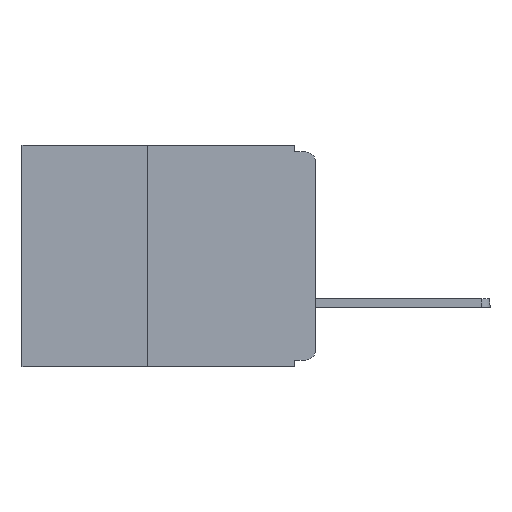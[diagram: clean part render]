
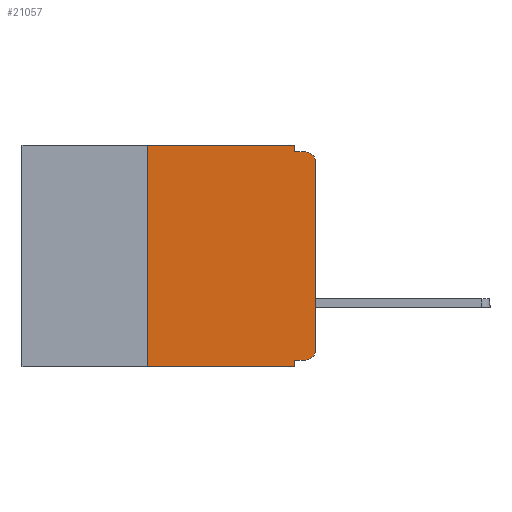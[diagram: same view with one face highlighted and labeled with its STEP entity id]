
A CAD part, left-side view. The second image highlights one B-rep face of the part: STEP entity #21057.
In plain terms, the highlighted planar face has unit normal (-1, 0, 0).
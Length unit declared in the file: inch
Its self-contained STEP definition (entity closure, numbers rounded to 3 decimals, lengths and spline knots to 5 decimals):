
#361 = VECTOR ( 'NONE', #23522, 39.37008 ) ;
#464 = VECTOR ( 'NONE', #29746, 39.37008 ) ;
#555 = DIRECTION ( 'NONE',  ( 0., 0., -1. ) ) ;
#592 = LINE ( 'NONE', #11071, #14531 ) ;
#637 = AXIS2_PLACEMENT_3D ( 'NONE', #30799, #15090, #33387 ) ;
#917 = ORIENTED_EDGE ( 'NONE', *, *, #19872, .F. ) ;
#2514 = ORIENTED_EDGE ( 'NONE', *, *, #29880, .F. ) ;
#3425 = VERTEX_POINT ( 'NONE', #17039 ) ;
#4144 = EDGE_CURVE ( 'NONE', #6339, #31770, #23790, .T. ) ;
#4825 = CARTESIAN_POINT ( 'NONE',  ( 0., 0., -0.305 ) ) ;
#5319 = CARTESIAN_POINT ( 'NONE',  ( 0., 0.437, 0. ) ) ;
#5727 = VERTEX_POINT ( 'NONE', #18445 ) ;
#5897 = CARTESIAN_POINT ( 'NONE',  ( 0., 0.031, 0. ) ) ;
#6339 = VERTEX_POINT ( 'NONE', #23707 ) ;
#6454 = EDGE_CURVE ( 'NONE', #5727, #31805, #20805, .T. ) ;
#6858 = EDGE_LOOP ( 'NONE', ( #20339, #23493, #17405, #27583, #917, #2514, #21348, #10965, #12615, #20300 ) ) ;
#7331 = DIRECTION ( 'NONE',  ( 1., 0., 0. ) ) ;
#7677 = EDGE_CURVE ( 'NONE', #17097, #15814, #9293, .T. ) ;
#7737 = DIRECTION ( 'NONE',  ( 0., 0., 1. ) ) ;
#7818 = CARTESIAN_POINT ( 'NONE',  ( 0., 0.015, -0.305 ) ) ;
#8336 = EDGE_CURVE ( 'NONE', #17097, #5727, #10124, .T. ) ;
#9293 = CIRCLE ( 'NONE', #22206, 0.015 ) ;
#9300 = VECTOR ( 'NONE', #18273, 39.37008 ) ;
#9304 = CARTESIAN_POINT ( 'NONE',  ( 0., 0.015, -0.32 ) ) ;
#9521 = VECTOR ( 'NONE', #12684, 39.37008 ) ;
#10124 = LINE ( 'NONE', #28785, #9300 ) ;
#10361 = VECTOR ( 'NONE', #14296, 39.37008 ) ;
#10410 = CARTESIAN_POINT ( 'NONE',  ( 0., 0.031, -0.33 ) ) ;
#10469 = DIRECTION ( 'NONE',  ( 0., 0., -1. ) ) ;
#10944 = EDGE_CURVE ( 'NONE', #15395, #16290, #21357, .T. ) ;
#10961 = DIRECTION ( 'NONE',  ( 0., -1., 0. ) ) ;
#10965 = ORIENTED_EDGE ( 'NONE', *, *, #6454, .F. ) ;
#11071 = CARTESIAN_POINT ( 'NONE',  ( 0., 0.437, -0.33 ) ) ;
#11640 = CARTESIAN_POINT ( 'NONE',  ( 0., 0., -0.01 ) ) ;
#12364 = PLANE ( 'NONE',  #29291 ) ;
#12502 = EDGE_CURVE ( 'NONE', #15814, #6339, #31156, .T. ) ;
#12615 = ORIENTED_EDGE ( 'NONE', *, *, #8336, .F. ) ;
#12684 = DIRECTION ( 'NONE',  ( 0., 0., 1. ) ) ;
#14296 = DIRECTION ( 'NONE',  ( 0., -1., 0. ) ) ;
#14316 = LINE ( 'NONE', #5319, #361 ) ;
#14531 = VECTOR ( 'NONE', #10961, 39.37008 ) ;
#14681 = VECTOR ( 'NONE', #555, 39.37008 ) ;
#14810 = LINE ( 'NONE', #31007, #9521 ) ;
#15090 = DIRECTION ( 'NONE',  ( -1., 0., 0. ) ) ;
#15109 = CARTESIAN_POINT ( 'NONE',  ( 0., 0.437, 0. ) ) ;
#15395 = VERTEX_POINT ( 'NONE', #5897 ) ;
#15814 = VERTEX_POINT ( 'NONE', #4825 ) ;
#15842 = FACE_OUTER_BOUND ( 'NONE', #6858, .T. ) ;
#16230 = CARTESIAN_POINT ( 'NONE',  ( 0., 0.031, -0.33 ) ) ;
#16290 = VERTEX_POINT ( 'NONE', #31330 ) ;
#17039 = CARTESIAN_POINT ( 'NONE',  ( 0., 0.25, -0.33 ) ) ;
#17097 = VERTEX_POINT ( 'NONE', #9304 ) ;
#17405 = ORIENTED_EDGE ( 'NONE', *, *, #29638, .F. ) ;
#18273 = DIRECTION ( 'NONE',  ( 0., 1., 0. ) ) ;
#18445 = CARTESIAN_POINT ( 'NONE',  ( 0., 0.031, -0.32 ) ) ;
#19210 = CARTESIAN_POINT ( 'NONE',  ( 0., 0.25, 0. ) ) ;
#19872 = EDGE_CURVE ( 'NONE', #21961, #15395, #14316, .T. ) ;
#20300 = ORIENTED_EDGE ( 'NONE', *, *, #7677, .T. ) ;
#20339 = ORIENTED_EDGE ( 'NONE', *, *, #12502, .T. ) ;
#20805 = LINE ( 'NONE', #16230, #14681 ) ;
#21057 = ADVANCED_FACE ( 'NONE', ( #15842 ), #12364, .F. ) ;
#21348 = ORIENTED_EDGE ( 'NONE', *, *, #28173, .T. ) ;
#21357 = LINE ( 'NONE', #24431, #464 ) ;
#21961 = VERTEX_POINT ( 'NONE', #19210 ) ;
#22206 = AXIS2_PLACEMENT_3D ( 'NONE', #7818, #26158, #10469 ) ;
#23493 = ORIENTED_EDGE ( 'NONE', *, *, #4144, .T. ) ;
#23522 = DIRECTION ( 'NONE',  ( 0., -1., 0. ) ) ;
#23707 = CARTESIAN_POINT ( 'NONE',  ( 0., 0., -0.025 ) ) ;
#23790 = CIRCLE ( 'NONE', #637, 0.015 ) ;
#24260 = LINE ( 'NONE', #11640, #10361 ) ;
#24431 = CARTESIAN_POINT ( 'NONE',  ( 0., 0.031, 0. ) ) ;
#25620 = DIRECTION ( 'NONE',  ( 0., 0., -1. ) ) ;
#26158 = DIRECTION ( 'NONE',  ( -1., 0., 0. ) ) ;
#27583 = ORIENTED_EDGE ( 'NONE', *, *, #10944, .F. ) ;
#28173 = EDGE_CURVE ( 'NONE', #3425, #31805, #592, .T. ) ;
#28530 = CARTESIAN_POINT ( 'NONE',  ( 0., 0.015, -0.01 ) ) ;
#28628 = CARTESIAN_POINT ( 'NONE',  ( 0., 0., 0. ) ) ;
#28785 = CARTESIAN_POINT ( 'NONE',  ( 0., 0., -0.32 ) ) ;
#29291 = AXIS2_PLACEMENT_3D ( 'NONE', #15109, #7331, #25620 ) ;
#29638 = EDGE_CURVE ( 'NONE', #16290, #31770, #24260, .T. ) ;
#29746 = DIRECTION ( 'NONE',  ( 0., 0., -1. ) ) ;
#29880 = EDGE_CURVE ( 'NONE', #3425, #21961, #14810, .T. ) ;
#30799 = CARTESIAN_POINT ( 'NONE',  ( 0., 0.015, -0.025 ) ) ;
#31007 = CARTESIAN_POINT ( 'NONE',  ( 0., 0.25, -0.33 ) ) ;
#31156 = LINE ( 'NONE', #28628, #31992 ) ;
#31330 = CARTESIAN_POINT ( 'NONE',  ( 0., 0.031, -0.01 ) ) ;
#31770 = VERTEX_POINT ( 'NONE', #28530 ) ;
#31805 = VERTEX_POINT ( 'NONE', #10410 ) ;
#31992 = VECTOR ( 'NONE', #7737, 39.37008 ) ;
#33387 = DIRECTION ( 'NONE',  ( 0., 0., -1. ) ) ;
